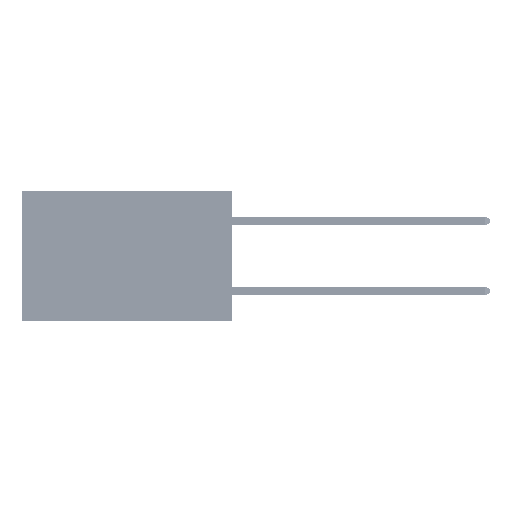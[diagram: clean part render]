
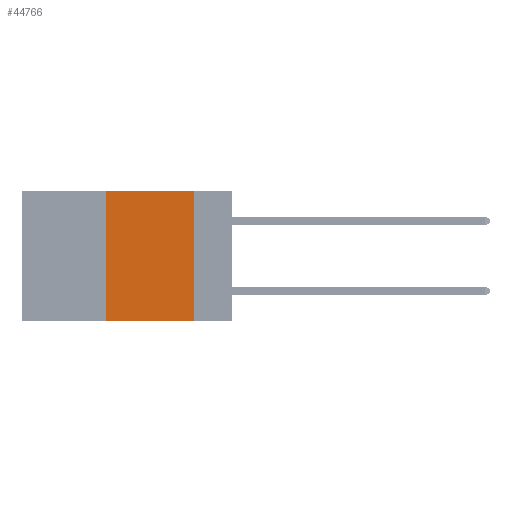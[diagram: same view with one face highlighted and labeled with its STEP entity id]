
A CAD part, left-side view. The second image highlights one B-rep face of the part: STEP entity #44766.
In plain terms, the highlighted planar face has unit normal (-1, 0, 0).
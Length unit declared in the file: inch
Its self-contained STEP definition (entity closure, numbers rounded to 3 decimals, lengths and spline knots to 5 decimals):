
#217 = AXIS2_PLACEMENT_3D ( 'NONE', #45836, #21763, #882 ) ;
#365 = CARTESIAN_POINT ( 'NONE',  ( 0., 0.11, -0.37 ) ) ;
#644 = ORIENTED_EDGE ( 'NONE', *, *, #34375, .F. ) ;
#882 = DIRECTION ( 'NONE',  ( 0., 0., -1. ) ) ;
#1101 = DIRECTION ( 'NONE',  ( 0., -1., 0. ) ) ;
#4668 = EDGE_CURVE ( 'NONE', #6148, #44676, #40461, .T. ) ;
#6148 = VERTEX_POINT ( 'NONE', #42824 ) ;
#9053 = EDGE_CURVE ( 'NONE', #6148, #27260, #24071, .T. ) ;
#9798 = LINE ( 'NONE', #41622, #14165 ) ;
#11471 = CARTESIAN_POINT ( 'NONE',  ( 0., 0.36, 0. ) ) ;
#11521 = LINE ( 'NONE', #23814, #38918 ) ;
#12036 = DIRECTION ( 'NONE',  ( 0., 0., 1. ) ) ;
#12792 = ORIENTED_EDGE ( 'NONE', *, *, #34956, .F. ) ;
#14165 = VECTOR ( 'NONE', #46702, 39.37008 ) ;
#21763 = DIRECTION ( 'NONE',  ( 1., 0., 0. ) ) ;
#23814 = CARTESIAN_POINT ( 'NONE',  ( 0., 0.11, 0. ) ) ;
#24071 = LINE ( 'NONE', #44905, #24894 ) ;
#24894 = VECTOR ( 'NONE', #12036, 39.37008 ) ;
#25098 = ORIENTED_EDGE ( 'NONE', *, *, #9053, .F. ) ;
#25852 = VECTOR ( 'NONE', #1101, 39.37008 ) ;
#27260 = VERTEX_POINT ( 'NONE', #11471 ) ;
#27947 = EDGE_LOOP ( 'NONE', ( #12792, #644, #25098, #52262 ) ) ;
#30040 = PLANE ( 'NONE',  #217 ) ;
#34375 = EDGE_CURVE ( 'NONE', #27260, #44731, #9798, .T. ) ;
#34956 = EDGE_CURVE ( 'NONE', #44731, #44676, #11521, .T. ) ;
#36374 = DIRECTION ( 'NONE',  ( 0., 0., -1. ) ) ;
#38918 = VECTOR ( 'NONE', #36374, 39.37008 ) ;
#40461 = LINE ( 'NONE', #47969, #25852 ) ;
#41547 = FACE_OUTER_BOUND ( 'NONE', #27947, .T. ) ;
#41622 = CARTESIAN_POINT ( 'NONE',  ( 0., 0.6, 0. ) ) ;
#42824 = CARTESIAN_POINT ( 'NONE',  ( 0., 0.36, -0.37 ) ) ;
#44676 = VERTEX_POINT ( 'NONE', #365 ) ;
#44731 = VERTEX_POINT ( 'NONE', #50115 ) ;
#44766 = ADVANCED_FACE ( 'NONE', ( #41547 ), #30040, .F. ) ;
#44905 = CARTESIAN_POINT ( 'NONE',  ( 0., 0.36, 0. ) ) ;
#45836 = CARTESIAN_POINT ( 'NONE',  ( 0., 0.6, 0. ) ) ;
#46702 = DIRECTION ( 'NONE',  ( 0., -1., 0. ) ) ;
#47969 = CARTESIAN_POINT ( 'NONE',  ( 0., 0.6, -0.37 ) ) ;
#50115 = CARTESIAN_POINT ( 'NONE',  ( 0., 0.11, 0. ) ) ;
#52262 = ORIENTED_EDGE ( 'NONE', *, *, #4668, .T. ) ;
